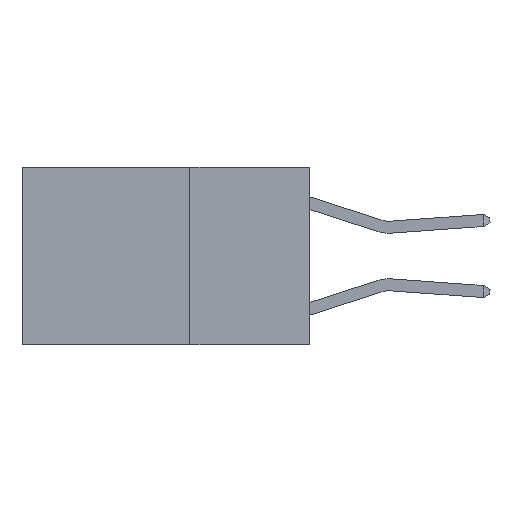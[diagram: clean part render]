
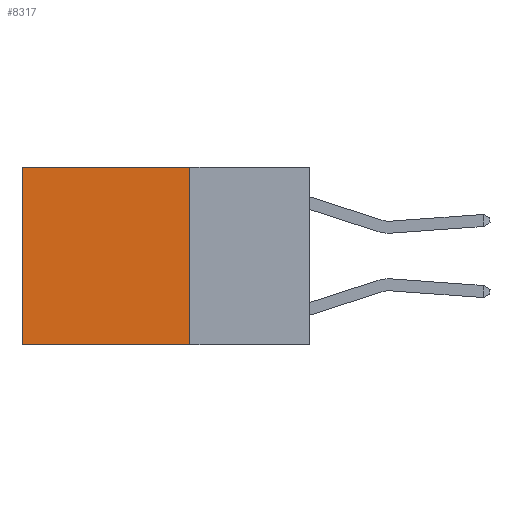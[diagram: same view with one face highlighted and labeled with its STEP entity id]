
A CAD part, left-side view. The second image highlights one B-rep face of the part: STEP entity #8317.
In plain terms, the highlighted planar face has unit normal (-1, 0, 0).
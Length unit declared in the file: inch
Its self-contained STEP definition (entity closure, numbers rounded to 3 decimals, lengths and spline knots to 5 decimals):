
#186 = VECTOR ( 'NONE', #3270, 39.37008 ) ;
#244 = EDGE_CURVE ( 'NONE', #795, #6283, #3883, .T. ) ;
#258 = VECTOR ( 'NONE', #5557, 39.37008 ) ;
#786 = ORIENTED_EDGE ( 'NONE', *, *, #1535, .T. ) ;
#795 = VERTEX_POINT ( 'NONE', #9383 ) ;
#1535 = EDGE_CURVE ( 'NONE', #5367, #7831, #2617, .T. ) ;
#1795 = DIRECTION ( 'NONE',  ( 0., 0., -1. ) ) ;
#1899 = CARTESIAN_POINT ( 'NONE',  ( 0.2625, 0.25, 0. ) ) ;
#2447 = EDGE_CURVE ( 'NONE', #5367, #795, #8452, .T. ) ;
#2617 = LINE ( 'NONE', #9741, #6457 ) ;
#2671 = DIRECTION ( 'NONE',  ( 0., 0., -1. ) ) ;
#3259 = CARTESIAN_POINT ( 'NONE',  ( 0.2625, 0.25, -0.37 ) ) ;
#3270 = DIRECTION ( 'NONE',  ( 0., 1., 0. ) ) ;
#3607 = AXIS2_PLACEMENT_3D ( 'NONE', #1899, #7237, #2671 ) ;
#3883 = LINE ( 'NONE', #3259, #186 ) ;
#4866 = ORIENTED_EDGE ( 'NONE', *, *, #244, .F. ) ;
#4883 = CARTESIAN_POINT ( 'NONE',  ( 0.2625, 0.6, 0. ) ) ;
#4897 = FACE_OUTER_BOUND ( 'NONE', #7613, .T. ) ;
#5265 = DIRECTION ( 'NONE',  ( 0., 1., 0. ) ) ;
#5367 = VERTEX_POINT ( 'NONE', #8886 ) ;
#5370 = VECTOR ( 'NONE', #1795, 39.37008 ) ;
#5443 = CARTESIAN_POINT ( 'NONE',  ( 0.2625, 0.6, -0.37 ) ) ;
#5557 = DIRECTION ( 'NONE',  ( 0., 0., -1. ) ) ;
#5850 = CARTESIAN_POINT ( 'NONE',  ( 0.2625, 0.6, 0. ) ) ;
#6283 = VERTEX_POINT ( 'NONE', #5443 ) ;
#6456 = ORIENTED_EDGE ( 'NONE', *, *, #8251, .T. ) ;
#6457 = VECTOR ( 'NONE', #5265, 39.37008 ) ;
#6495 = PLANE ( 'NONE',  #3607 ) ;
#7237 = DIRECTION ( 'NONE',  ( 1., 0., 0. ) ) ;
#7349 = LINE ( 'NONE', #4883, #5370 ) ;
#7613 = EDGE_LOOP ( 'NONE', ( #6456, #4866, #8772, #786 ) ) ;
#7831 = VERTEX_POINT ( 'NONE', #5850 ) ;
#8251 = EDGE_CURVE ( 'NONE', #7831, #6283, #7349, .T. ) ;
#8317 = ADVANCED_FACE ( 'NONE', ( #4897 ), #6495, .F. ) ;
#8452 = LINE ( 'NONE', #9288, #258 ) ;
#8772 = ORIENTED_EDGE ( 'NONE', *, *, #2447, .F. ) ;
#8886 = CARTESIAN_POINT ( 'NONE',  ( 0.2625, 0.25, 0. ) ) ;
#9288 = CARTESIAN_POINT ( 'NONE',  ( 0.2625, 0.25, 0. ) ) ;
#9383 = CARTESIAN_POINT ( 'NONE',  ( 0.2625, 0.25, -0.37 ) ) ;
#9741 = CARTESIAN_POINT ( 'NONE',  ( 0.2625, 0.25, 0. ) ) ;
